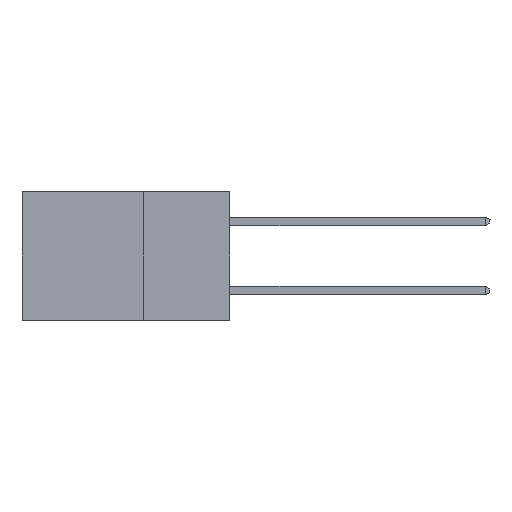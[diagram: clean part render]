
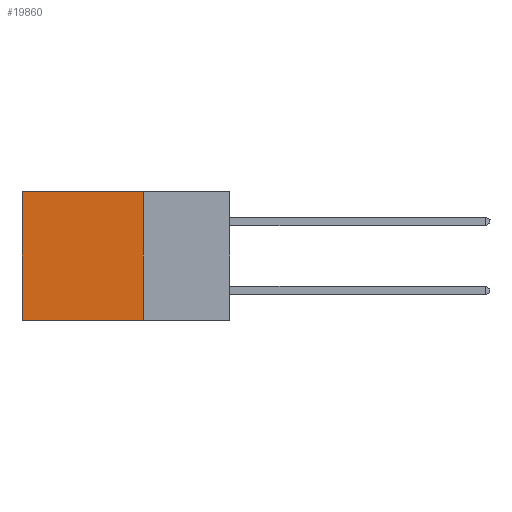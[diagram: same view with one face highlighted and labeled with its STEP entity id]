
A CAD part, left-side view. The second image highlights one B-rep face of the part: STEP entity #19860.
In plain terms, the highlighted planar face has unit normal (-1, 0, 0).
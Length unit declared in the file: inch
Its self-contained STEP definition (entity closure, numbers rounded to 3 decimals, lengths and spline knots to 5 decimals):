
#395 = CARTESIAN_POINT ( 'NONE',  ( 0.298, 0.6, 0. ) ) ;
#1184 = CARTESIAN_POINT ( 'NONE',  ( 0.298, 0.6, 0. ) ) ;
#1994 = ORIENTED_EDGE ( 'NONE', *, *, #6183, .T. ) ;
#2053 = ORIENTED_EDGE ( 'NONE', *, *, #5119, .F. ) ;
#4213 = VECTOR ( 'NONE', #10056, 39.37008 ) ;
#4646 = LINE ( 'NONE', #1184, #15329 ) ;
#5119 = EDGE_CURVE ( 'NONE', #21304, #16204, #26813, .T. ) ;
#5729 = VERTEX_POINT ( 'NONE', #10521 ) ;
#6183 = EDGE_CURVE ( 'NONE', #5729, #6377, #11443, .T. ) ;
#6377 = VERTEX_POINT ( 'NONE', #395 ) ;
#7099 = VECTOR ( 'NONE', #14014, 39.37008 ) ;
#7226 = CARTESIAN_POINT ( 'NONE',  ( 0.298, 0.25, 0. ) ) ;
#7780 = ORIENTED_EDGE ( 'NONE', *, *, #9307, .F. ) ;
#9307 = EDGE_CURVE ( 'NONE', #5729, #21304, #15573, .T. ) ;
#9376 = DIRECTION ( 'NONE',  ( 1., 0., 0. ) ) ;
#9847 = VECTOR ( 'NONE', #23447, 39.37008 ) ;
#10056 = DIRECTION ( 'NONE',  ( 0., 0., -1. ) ) ;
#10314 = ORIENTED_EDGE ( 'NONE', *, *, #21821, .T. ) ;
#10521 = CARTESIAN_POINT ( 'NONE',  ( 0.298, 0.25, 0. ) ) ;
#11443 = LINE ( 'NONE', #24603, #7099 ) ;
#12881 = CARTESIAN_POINT ( 'NONE',  ( 0.298, 0.6, -0.37 ) ) ;
#14014 = DIRECTION ( 'NONE',  ( 0., 1., 0. ) ) ;
#14071 = EDGE_LOOP ( 'NONE', ( #10314, #2053, #7780, #1994 ) ) ;
#14236 = CARTESIAN_POINT ( 'NONE',  ( 0.298, 0.25, 0. ) ) ;
#14365 = FACE_OUTER_BOUND ( 'NONE', #14071, .T. ) ;
#15329 = VECTOR ( 'NONE', #22453, 39.37008 ) ;
#15573 = LINE ( 'NONE', #14236, #4213 ) ;
#16204 = VERTEX_POINT ( 'NONE', #12881 ) ;
#17296 = AXIS2_PLACEMENT_3D ( 'NONE', #7226, #9376, #24238 ) ;
#19860 = ADVANCED_FACE ( 'NONE', ( #14365 ), #19956, .F. ) ;
#19956 = PLANE ( 'NONE',  #17296 ) ;
#20830 = CARTESIAN_POINT ( 'NONE',  ( 0.298, 0.25, -0.37 ) ) ;
#21303 = CARTESIAN_POINT ( 'NONE',  ( 0.298, 0.25, -0.37 ) ) ;
#21304 = VERTEX_POINT ( 'NONE', #20830 ) ;
#21821 = EDGE_CURVE ( 'NONE', #6377, #16204, #4646, .T. ) ;
#22453 = DIRECTION ( 'NONE',  ( 0., 0., -1. ) ) ;
#23447 = DIRECTION ( 'NONE',  ( 0., 1., 0. ) ) ;
#24238 = DIRECTION ( 'NONE',  ( 0., 0., -1. ) ) ;
#24603 = CARTESIAN_POINT ( 'NONE',  ( 0.298, 0.25, 0. ) ) ;
#26813 = LINE ( 'NONE', #21303, #9847 ) ;
